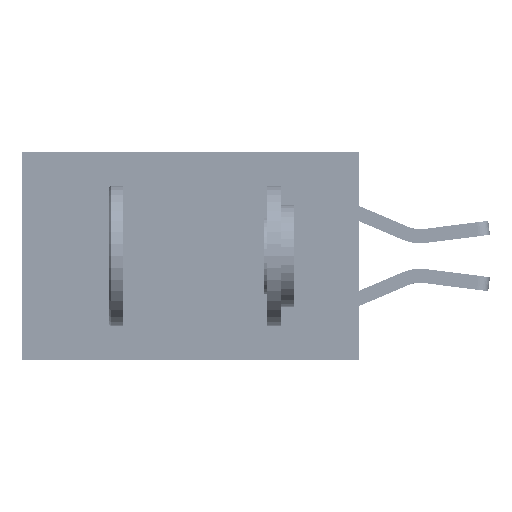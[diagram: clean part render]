
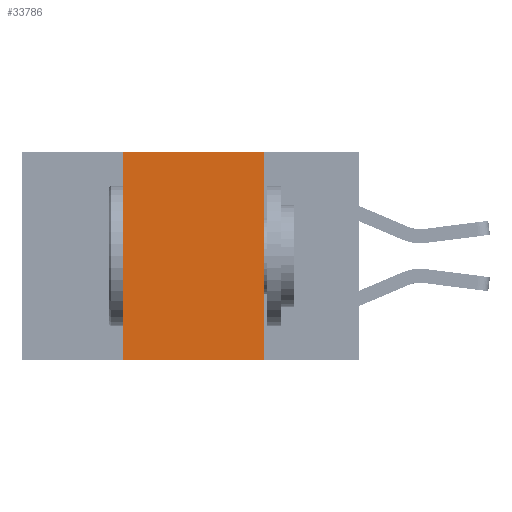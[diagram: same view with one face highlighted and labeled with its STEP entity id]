
A CAD part, left-side view. The second image highlights one B-rep face of the part: STEP entity #33786.
In plain terms, the highlighted planar face has unit normal (-1, 0, 0).
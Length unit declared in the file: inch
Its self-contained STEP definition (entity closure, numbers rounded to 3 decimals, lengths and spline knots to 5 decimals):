
#1100 = EDGE_CURVE ( 'NONE', #26857, #42385, #37903, .T. ) ;
#1950 = EDGE_CURVE ( 'NONE', #42385, #30343, #17403, .T. ) ;
#3945 = CARTESIAN_POINT ( 'NONE',  ( 0., 0.42, -0.37 ) ) ;
#5588 = DIRECTION ( 'NONE',  ( 0., -1., 0. ) ) ;
#9341 = VECTOR ( 'NONE', #10770, 39.37008 ) ;
#10770 = DIRECTION ( 'NONE',  ( 0., -1., 0. ) ) ;
#10842 = ORIENTED_EDGE ( 'NONE', *, *, #20085, .T. ) ;
#12274 = LINE ( 'NONE', #18479, #9341 ) ;
#14472 = CARTESIAN_POINT ( 'NONE',  ( 0., 0.42, 0. ) ) ;
#14974 = DIRECTION ( 'NONE',  ( 0., 0., -1. ) ) ;
#14988 = DIRECTION ( 'NONE',  ( 0., 0., -1. ) ) ;
#16848 = VECTOR ( 'NONE', #5588, 39.37008 ) ;
#17403 = LINE ( 'NONE', #35790, #16848 ) ;
#17477 = DIRECTION ( 'NONE',  ( 0., 0., 1. ) ) ;
#18479 = CARTESIAN_POINT ( 'NONE',  ( 0., 0.6, -0.37 ) ) ;
#20085 = EDGE_CURVE ( 'NONE', #26857, #23286, #12274, .T. ) ;
#20333 = FACE_OUTER_BOUND ( 'NONE', #46025, .T. ) ;
#21527 = ORIENTED_EDGE ( 'NONE', *, *, #1950, .F. ) ;
#21605 = PLANE ( 'NONE',  #39335 ) ;
#23286 = VERTEX_POINT ( 'NONE', #29140 ) ;
#24321 = CARTESIAN_POINT ( 'NONE',  ( 0., 0.17, 0. ) ) ;
#26857 = VERTEX_POINT ( 'NONE', #3945 ) ;
#29140 = CARTESIAN_POINT ( 'NONE',  ( 0., 0.17, -0.37 ) ) ;
#30119 = LINE ( 'NONE', #41058, #33598 ) ;
#30164 = ORIENTED_EDGE ( 'NONE', *, *, #1100, .F. ) ;
#30343 = VERTEX_POINT ( 'NONE', #24321 ) ;
#30699 = EDGE_CURVE ( 'NONE', #30343, #23286, #30119, .T. ) ;
#33598 = VECTOR ( 'NONE', #14974, 39.37008 ) ;
#33786 = ADVANCED_FACE ( 'NONE', ( #20333 ), #21605, .F. ) ;
#35790 = CARTESIAN_POINT ( 'NONE',  ( 0., 0.6, 0. ) ) ;
#37903 = LINE ( 'NONE', #48010, #44308 ) ;
#39335 = AXIS2_PLACEMENT_3D ( 'NONE', #47687, #45163, #14988 ) ;
#41058 = CARTESIAN_POINT ( 'NONE',  ( 0., 0.17, 0. ) ) ;
#42385 = VERTEX_POINT ( 'NONE', #14472 ) ;
#44308 = VECTOR ( 'NONE', #17477, 39.37008 ) ;
#45163 = DIRECTION ( 'NONE',  ( 1., 0., 0. ) ) ;
#46025 = EDGE_LOOP ( 'NONE', ( #47553, #21527, #30164, #10842 ) ) ;
#47553 = ORIENTED_EDGE ( 'NONE', *, *, #30699, .F. ) ;
#47687 = CARTESIAN_POINT ( 'NONE',  ( 0., 0.6, 0. ) ) ;
#48010 = CARTESIAN_POINT ( 'NONE',  ( 0., 0.42, 0. ) ) ;
